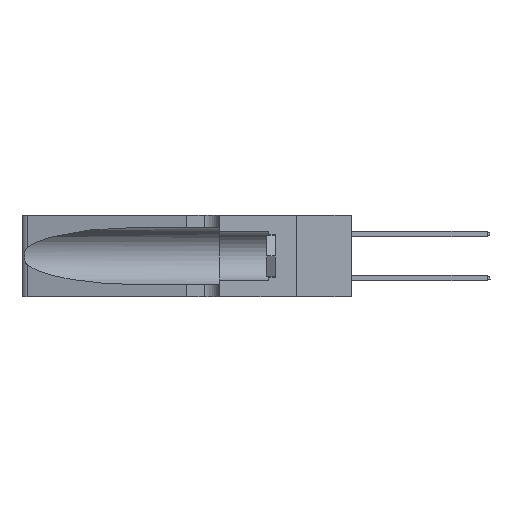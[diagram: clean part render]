
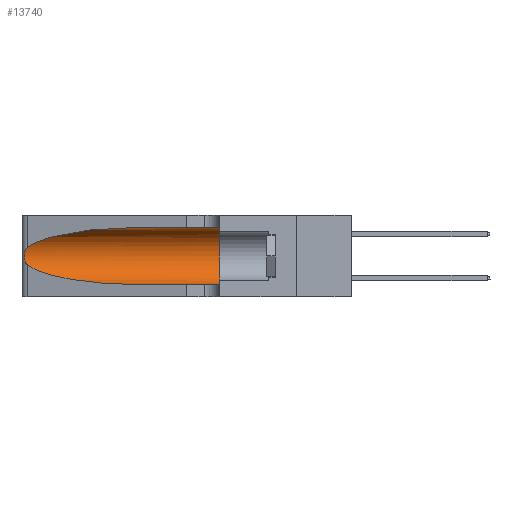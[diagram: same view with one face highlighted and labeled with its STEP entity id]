
A CAD part, left-side view. The second image highlights one B-rep face of the part: STEP entity #13740.
In plain terms, the highlighted cylindrical face has radius 3.308 mm (diameter 6.617 mm), a partial arc.
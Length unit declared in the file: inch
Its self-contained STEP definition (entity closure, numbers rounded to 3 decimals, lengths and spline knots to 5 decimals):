
#1091 = CYLINDRICAL_SURFACE ( 'NONE', #21812, 0.13025 ) ;
#1538 = CARTESIAN_POINT ( 'NONE',  ( 0.1305, 0.72297, 0.31525 ) ) ;
#1545 = DIRECTION ( 'NONE',  ( 0., -1., 0. ) ) ;
#2086 = CARTESIAN_POINT ( 'NONE',  ( 0.25639, 1.23184, 0.21858 ) ) ;
#2785 = EDGE_CURVE ( 'NONE', #30908, #6223, #29092, .T. ) ;
#3095 = CARTESIAN_POINT ( 'NONE',  ( 0.1305, 0.35, 0.185 ) ) ;
#4021 = ORIENTED_EDGE ( 'NONE', *, *, #40803, .F. ) ;
#4364 = VERTEX_POINT ( 'NONE', #1538 ) ;
#5845 = CARTESIAN_POINT ( 'NONE',  ( 0.25787, 1.23484, 0.2124 ) ) ;
#6223 = VERTEX_POINT ( 'NONE', #34511 ) ;
#6310 = FACE_OUTER_BOUND ( 'NONE', #30305, .T. ) ;
#6396 = CARTESIAN_POINT ( 'NONE',  ( 0.2373, 1.15595, 0.28018 ) ) ;
#7440 = CARTESIAN_POINT ( 'NONE',  ( 0.25487, 1.22718, 0.14631 ) ) ;
#8336 = EDGE_CURVE ( 'NONE', #14460, #6223, #25026, .T. ) ;
#8400 = CARTESIAN_POINT ( 'NONE',  ( 0.25487, 1.22718, 0.22369 ) ) ;
#8721 = CARTESIAN_POINT ( 'NONE',  ( 0.25487, 1.22718, 0.22369 ) ) ;
#9286 = CARTESIAN_POINT ( 'NONE',  ( 0.18966, 0.96281, 0.31525 ) ) ;
#10012 = AXIS2_PLACEMENT_3D ( 'NONE', #3095, #32977, #13292 ) ;
#10190 = CARTESIAN_POINT ( 'NONE',  ( 0.1305, 0.35, 0.31525 ) ) ;
#10444 = ORIENTED_EDGE ( 'NONE', *, *, #31832, .T. ) ;
#11100 = CARTESIAN_POINT ( 'NONE',  ( 0.1305, 1.61858, 0.05475 ) ) ;
#12333 = CARTESIAN_POINT ( 'NONE',  ( 0.25487, 1.22718, 0.14631 ) ) ;
#12870 = CARTESIAN_POINT ( 'NONE',  ( 0.25487, 1.22718, 0.22369 ) ) ;
#13004 = CARTESIAN_POINT ( 'NONE',  ( 0.1305, 0.72297, 0.31525 ) ) ;
#13292 = DIRECTION ( 'NONE',  ( 0., 0., 1. ) ) ;
#13729 = EDGE_CURVE ( 'NONE', #25253, #14460, #13902, .T. ) ;
#13740 = ADVANCED_FACE ( 'NONE', ( #6310 ), #1091, .F. ) ;
#13902 =( BOUNDED_CURVE ( )  B_SPLINE_CURVE ( 3, ( #7440, #33618, #36865, #28248 ),
 .UNSPECIFIED., .F., .T. ) 
 B_SPLINE_CURVE_WITH_KNOTS ( ( 4, 4 ),
 ( 3.44316, 4.71239 ),
 .UNSPECIFIED. ) 
 CURVE ( )  GEOMETRIC_REPRESENTATION_ITEM ( )  RATIONAL_B_SPLINE_CURVE ( ( 1., 0.87, 0.87, 1. ) ) 
 REPRESENTATION_ITEM ( '' )  );
#14460 = VERTEX_POINT ( 'NONE', #22194 ) ;
#14565 = DIRECTION ( 'NONE',  ( 0., -1., 0. ) ) ;
#14582 = DIRECTION ( 'NONE',  ( 0., -1., 0. ) ) ;
#18384 = B_SPLINE_CURVE_WITH_KNOTS ( 'NONE', 3,
 ( #8721, #18757, #2086, #5845, #25195, #28761, #22031, #35418, #31748, #35288, #38129, #35018, #32017, #12333 ),
 .UNSPECIFIED., .F., .F.,
 ( 4, 2, 2, 2, 2, 2, 4 ),
 ( 0., 0.00027, 0.00053, 0.00107, 0.0016, 0.00187, 0.00214 ),
 .UNSPECIFIED. ) ;
#18757 = CARTESIAN_POINT ( 'NONE',  ( 0.25555, 1.22994, 0.2215 ) ) ;
#21812 = AXIS2_PLACEMENT_3D ( 'NONE', #38025, #1545, #37737 ) ;
#22031 = CARTESIAN_POINT ( 'NONE',  ( 0.26075, 1.23896, 0.19203 ) ) ;
#22194 = CARTESIAN_POINT ( 'NONE',  ( 0.1305, 0.72297, 0.05475 ) ) ;
#25026 = LINE ( 'NONE', #11100, #36703 ) ;
#25078 = VERTEX_POINT ( 'NONE', #8400 ) ;
#25195 = CARTESIAN_POINT ( 'NONE',  ( 0.25854, 1.2359, 0.20912 ) ) ;
#25253 = VERTEX_POINT ( 'NONE', #32117 ) ;
#25465 =( BOUNDED_CURVE ( )  B_SPLINE_CURVE ( 3, ( #13004, #9286, #6396, #12870 ),
 .UNSPECIFIED., .F., .F. ) 
 B_SPLINE_CURVE_WITH_KNOTS ( ( 4, 4 ),
 ( 1.5708, 2.84003 ),
 .UNSPECIFIED. ) 
 CURVE ( )  GEOMETRIC_REPRESENTATION_ITEM ( )  RATIONAL_B_SPLINE_CURVE ( ( 1., 0.87, 0.87, 1. ) ) 
 REPRESENTATION_ITEM ( '' )  );
#28248 = CARTESIAN_POINT ( 'NONE',  ( 0.1305, 0.72297, 0.05475 ) ) ;
#28761 = CARTESIAN_POINT ( 'NONE',  ( 0.26018, 1.23835, 0.19895 ) ) ;
#29092 = CIRCLE ( 'NONE', #10012, 0.13025 ) ;
#30305 = EDGE_LOOP ( 'NONE', ( #42145, #10444, #32030, #41028, #36845, #4021 ) ) ;
#30908 = VERTEX_POINT ( 'NONE', #10190 ) ;
#31748 = CARTESIAN_POINT ( 'NONE',  ( 0.26017, 1.23833, 0.17102 ) ) ;
#31832 = EDGE_CURVE ( 'NONE', #25078, #25253, #18384, .T. ) ;
#32017 = CARTESIAN_POINT ( 'NONE',  ( 0.25555, 1.22993, 0.14849 ) ) ;
#32030 = ORIENTED_EDGE ( 'NONE', *, *, #13729, .T. ) ;
#32117 = CARTESIAN_POINT ( 'NONE',  ( 0.25487, 1.22718, 0.14631 ) ) ;
#32144 = LINE ( 'NONE', #34116, #36673 ) ;
#32977 = DIRECTION ( 'NONE',  ( 0., 1., 0. ) ) ;
#33618 = CARTESIAN_POINT ( 'NONE',  ( 0.2373, 1.15595, 0.08982 ) ) ;
#33867 = EDGE_CURVE ( 'NONE', #4364, #25078, #25465, .T. ) ;
#34116 = CARTESIAN_POINT ( 'NONE',  ( 0.1305, 1.61858, 0.31525 ) ) ;
#34511 = CARTESIAN_POINT ( 'NONE',  ( 0.1305, 0.35, 0.05475 ) ) ;
#35018 = CARTESIAN_POINT ( 'NONE',  ( 0.25639, 1.23186, 0.15144 ) ) ;
#35288 = CARTESIAN_POINT ( 'NONE',  ( 0.25856, 1.23593, 0.16098 ) ) ;
#35418 = CARTESIAN_POINT ( 'NONE',  ( 0.26075, 1.23896, 0.178 ) ) ;
#36673 = VECTOR ( 'NONE', #14582, 39.37008 ) ;
#36703 = VECTOR ( 'NONE', #14565, 39.37008 ) ;
#36845 = ORIENTED_EDGE ( 'NONE', *, *, #2785, .F. ) ;
#36865 = CARTESIAN_POINT ( 'NONE',  ( 0.18966, 0.96281, 0.05475 ) ) ;
#37737 = DIRECTION ( 'NONE',  ( 0., 0., -1. ) ) ;
#38025 = CARTESIAN_POINT ( 'NONE',  ( 0.1305, 1.61858, 0.185 ) ) ;
#38129 = CARTESIAN_POINT ( 'NONE',  ( 0.25789, 1.23486, 0.15765 ) ) ;
#40803 = EDGE_CURVE ( 'NONE', #4364, #30908, #32144, .T. ) ;
#41028 = ORIENTED_EDGE ( 'NONE', *, *, #8336, .T. ) ;
#42145 = ORIENTED_EDGE ( 'NONE', *, *, #33867, .T. ) ;
